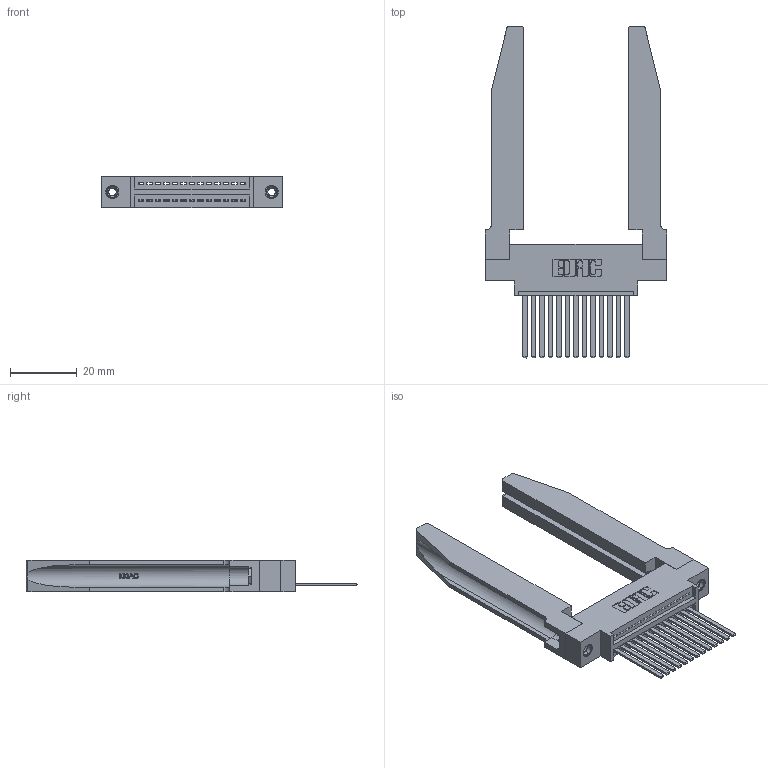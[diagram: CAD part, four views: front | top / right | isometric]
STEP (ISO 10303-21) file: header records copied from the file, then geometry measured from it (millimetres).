
FILE_DESCRIPTION (( 'STEP AP203' ), '1' );
FILE_NAME ('345-013-544-678.STEP', '2019-10-04T04:39:55', ( '' ), ( '' ), 'SwSTEP 2.0', 'SolidWorks 2016', '' );
FILE_SCHEMA (( 'CONFIG_CONTROL_DESIGN' ));
Length unit declared in the file: inch
Products named in the file (5): 345-220-078_345-220-078; 345-250-001_345-250-001-102; 345-013-544-678; 345-292-001_345-293-144; 345 Part_0.170 Offset - 0.156 Dia-TH
Assembly tree (18 placements, depth 2):
  345-013-544-678
    345 Part_0.170 Offset - 0.156 Dia-TH
    345-292-001_345-293-144  x13
    345-250-001_345-250-001-102  x2
    345-220-078_345-220-078  x2
Bounding box: 54.25 x 99.24 x 9.4 mm (x, y, z)
Volume: 12723.2 mm3; surface area: 13611.7 mm2
Topology: 18 solids, 18 shells, 1040 faces, 3015 edges, 1982 vertices
Faces by surface type: plane 694, cylinder 294, bspline 36, cone 12, torus 4
Entity records: 18376 total; most frequent: CARTESIAN_POINT 4082, ORIENTED_EDGE 2926, DIRECTION 2611, EDGE_CURVE 1463, VECTOR 1189, LINE 1189, VERTEX_POINT 968, AXIS2_PLACEMENT_3D 711
